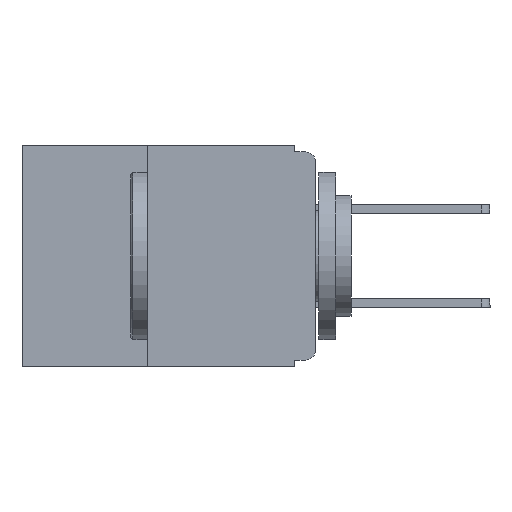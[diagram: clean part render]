
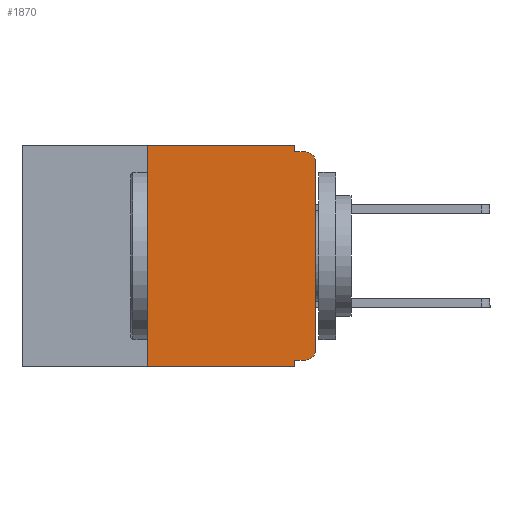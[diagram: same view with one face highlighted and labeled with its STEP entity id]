
A CAD part, left-side view. The second image highlights one B-rep face of the part: STEP entity #1870.
In plain terms, the highlighted planar face has unit normal (-1, 0, 0).
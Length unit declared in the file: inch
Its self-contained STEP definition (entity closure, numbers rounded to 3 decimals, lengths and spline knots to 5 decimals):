
#626 = VECTOR ( 'NONE', #17025, 39.37008 ) ;
#767 = DIRECTION ( 'NONE',  ( 0., 0., -1. ) ) ;
#881 = EDGE_CURVE ( 'NONE', #16906, #12202, #4911, .T. ) ;
#926 = ORIENTED_EDGE ( 'NONE', *, *, #22097, .T. ) ;
#1150 = ORIENTED_EDGE ( 'NONE', *, *, #8142, .T. ) ;
#1870 = ADVANCED_FACE ( 'NONE', ( #7861 ), #19893, .F. ) ;
#2214 = VECTOR ( 'NONE', #6678, 39.37008 ) ;
#2404 = VERTEX_POINT ( 'NONE', #5687 ) ;
#2443 = ORIENTED_EDGE ( 'NONE', *, *, #24829, .F. ) ;
#2683 = DIRECTION ( 'NONE',  ( 0., 0., -1. ) ) ;
#3295 = ORIENTED_EDGE ( 'NONE', *, *, #23080, .T. ) ;
#3625 = ORIENTED_EDGE ( 'NONE', *, *, #881, .F. ) ;
#3735 = CARTESIAN_POINT ( 'NONE',  ( 0., 0., -0.01 ) ) ;
#3758 = CARTESIAN_POINT ( 'NONE',  ( 0., 0.031, -0.01 ) ) ;
#4070 = LINE ( 'NONE', #26125, #9657 ) ;
#4234 = CARTESIAN_POINT ( 'NONE',  ( 0., 0.25, -0.33 ) ) ;
#4765 = AXIS2_PLACEMENT_3D ( 'NONE', #13157, #14969, #767 ) ;
#4911 = LINE ( 'NONE', #17169, #28266 ) ;
#4978 = EDGE_CURVE ( 'NONE', #12202, #23047, #25032, .T. ) ;
#5687 = CARTESIAN_POINT ( 'NONE',  ( 0., 0.25, 0. ) ) ;
#5766 = DIRECTION ( 'NONE',  ( -1., 0., 0. ) ) ;
#6216 = DIRECTION ( 'NONE',  ( 0., -1., 0. ) ) ;
#6246 = ORIENTED_EDGE ( 'NONE', *, *, #10553, .F. ) ;
#6678 = DIRECTION ( 'NONE',  ( 0., 0., 1. ) ) ;
#6951 = CARTESIAN_POINT ( 'NONE',  ( 0., 0., 0. ) ) ;
#7555 = VECTOR ( 'NONE', #23313, 39.37008 ) ;
#7694 = CARTESIAN_POINT ( 'NONE',  ( 0., 0., -0.025 ) ) ;
#7861 = FACE_OUTER_BOUND ( 'NONE', #24586, .T. ) ;
#8142 = EDGE_CURVE ( 'NONE', #15446, #23047, #16835, .T. ) ;
#8647 = LINE ( 'NONE', #4234, #2214 ) ;
#9657 = VECTOR ( 'NONE', #2683, 39.37008 ) ;
#10464 = CARTESIAN_POINT ( 'NONE',  ( 0., 0.015, -0.025 ) ) ;
#10536 = CARTESIAN_POINT ( 'NONE',  ( 0., 0.25, -0.33 ) ) ;
#10553 = EDGE_CURVE ( 'NONE', #23839, #17990, #29035, .T. ) ;
#10649 = VECTOR ( 'NONE', #24713, 39.37008 ) ;
#11322 = EDGE_CURVE ( 'NONE', #15446, #2404, #8647, .T. ) ;
#11407 = VERTEX_POINT ( 'NONE', #23345 ) ;
#12202 = VERTEX_POINT ( 'NONE', #13904 ) ;
#12833 = DIRECTION ( 'NONE',  ( 0., 0., -1. ) ) ;
#12858 = DIRECTION ( 'NONE',  ( 0., -1., 0. ) ) ;
#12900 = EDGE_CURVE ( 'NONE', #11407, #23839, #4070, .T. ) ;
#13157 = CARTESIAN_POINT ( 'NONE',  ( 0., 0.437, 0. ) ) ;
#13904 = CARTESIAN_POINT ( 'NONE',  ( 0., 0.031, -0.32 ) ) ;
#14810 = CARTESIAN_POINT ( 'NONE',  ( 0., 0.015, -0.01 ) ) ;
#14969 = DIRECTION ( 'NONE',  ( 1., 0., 0. ) ) ;
#15446 = VERTEX_POINT ( 'NONE', #10536 ) ;
#16123 = DIRECTION ( 'NONE',  ( 0., 1., 0. ) ) ;
#16367 = CARTESIAN_POINT ( 'NONE',  ( 0., 0., -0.305 ) ) ;
#16746 = AXIS2_PLACEMENT_3D ( 'NONE', #19803, #5766, #22142 ) ;
#16835 = LINE ( 'NONE', #24782, #10649 ) ;
#16906 = VERTEX_POINT ( 'NONE', #27139 ) ;
#17025 = DIRECTION ( 'NONE',  ( 0., 0., -1. ) ) ;
#17169 = CARTESIAN_POINT ( 'NONE',  ( 0., 0., -0.32 ) ) ;
#17188 = CARTESIAN_POINT ( 'NONE',  ( 0., 0.031, -0.33 ) ) ;
#17990 = VERTEX_POINT ( 'NONE', #14810 ) ;
#19019 = CIRCLE ( 'NONE', #27726, 0.015 ) ;
#19264 = LINE ( 'NONE', #6951, #7555 ) ;
#19709 = VERTEX_POINT ( 'NONE', #16367 ) ;
#19793 = CARTESIAN_POINT ( 'NONE',  ( 0., 0.437, 0. ) ) ;
#19803 = CARTESIAN_POINT ( 'NONE',  ( 0., 0.015, -0.305 ) ) ;
#19893 = PLANE ( 'NONE',  #4765 ) ;
#22097 = EDGE_CURVE ( 'NONE', #16906, #19709, #23314, .T. ) ;
#22142 = DIRECTION ( 'NONE',  ( 0., 0., -1. ) ) ;
#22904 = ORIENTED_EDGE ( 'NONE', *, *, #26725, .T. ) ;
#22985 = VECTOR ( 'NONE', #6216, 39.37008 ) ;
#23047 = VERTEX_POINT ( 'NONE', #27714 ) ;
#23080 = EDGE_CURVE ( 'NONE', #19709, #29402, #19264, .T. ) ;
#23313 = DIRECTION ( 'NONE',  ( 0., 0., 1. ) ) ;
#23314 = CIRCLE ( 'NONE', #16746, 0.015 ) ;
#23345 = CARTESIAN_POINT ( 'NONE',  ( 0., 0.031, 0. ) ) ;
#23513 = LINE ( 'NONE', #19793, #28858 ) ;
#23839 = VERTEX_POINT ( 'NONE', #3758 ) ;
#24110 = ORIENTED_EDGE ( 'NONE', *, *, #12900, .F. ) ;
#24586 = EDGE_LOOP ( 'NONE', ( #3295, #22904, #6246, #24110, #2443, #27954, #1150, #28726, #3625, #926 ) ) ;
#24713 = DIRECTION ( 'NONE',  ( 0., -1., 0. ) ) ;
#24782 = CARTESIAN_POINT ( 'NONE',  ( 0., 0.437, -0.33 ) ) ;
#24829 = EDGE_CURVE ( 'NONE', #2404, #11407, #23513, .T. ) ;
#25032 = LINE ( 'NONE', #17188, #626 ) ;
#26125 = CARTESIAN_POINT ( 'NONE',  ( 0., 0.031, 0. ) ) ;
#26725 = EDGE_CURVE ( 'NONE', #29402, #17990, #19019, .T. ) ;
#26737 = DIRECTION ( 'NONE',  ( -1., 0., 0. ) ) ;
#27139 = CARTESIAN_POINT ( 'NONE',  ( 0., 0.015, -0.32 ) ) ;
#27714 = CARTESIAN_POINT ( 'NONE',  ( 0., 0.031, -0.33 ) ) ;
#27726 = AXIS2_PLACEMENT_3D ( 'NONE', #10464, #26737, #12833 ) ;
#27954 = ORIENTED_EDGE ( 'NONE', *, *, #11322, .F. ) ;
#28266 = VECTOR ( 'NONE', #16123, 39.37008 ) ;
#28726 = ORIENTED_EDGE ( 'NONE', *, *, #4978, .F. ) ;
#28858 = VECTOR ( 'NONE', #12858, 39.37008 ) ;
#29035 = LINE ( 'NONE', #3735, #22985 ) ;
#29402 = VERTEX_POINT ( 'NONE', #7694 ) ;
